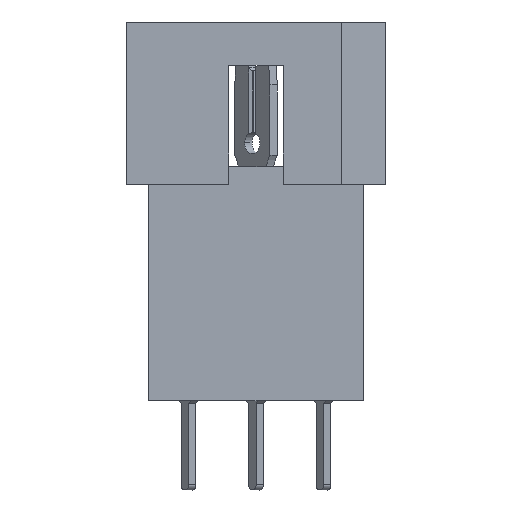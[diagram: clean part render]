
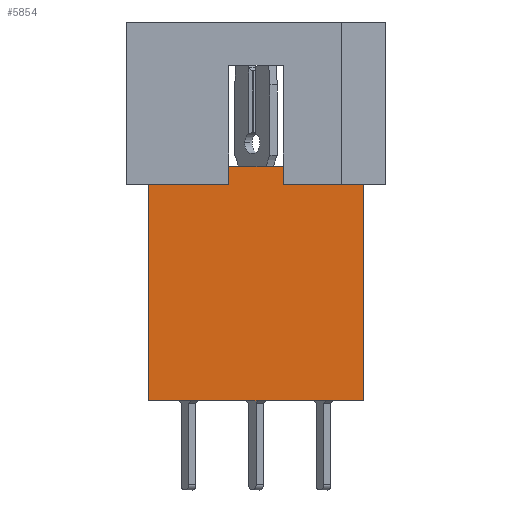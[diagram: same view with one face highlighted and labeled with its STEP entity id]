
A CAD part, top view. The second image highlights one B-rep face of the part: STEP entity #5854.
In plain terms, the highlighted planar face has unit normal (0, 0, 1).
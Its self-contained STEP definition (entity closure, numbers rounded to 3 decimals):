
#20 = CARTESIAN_POINT ( 'NONE',  ( 5.563, 0., 2.54 ) ) ;
#163 = DIRECTION ( 'NONE',  ( 1., 0., 0. ) ) ;
#215 = VECTOR ( 'NONE', #2633, 1000. ) ;
#218 = VECTOR ( 'NONE', #1200, 1000. ) ;
#232 = EDGE_LOOP ( 'NONE', ( #4984, #563, #6303, #2303, #3558, #2815, #1985, #5586 ) ) ;
#261 = VECTOR ( 'NONE', #4432, 1000. ) ;
#319 = CARTESIAN_POINT ( 'NONE',  ( -2.324, 0., 2.54 ) ) ;
#379 = LINE ( 'NONE', #5219, #218 ) ;
#386 = VERTEX_POINT ( 'NONE', #4853 ) ;
#469 = DIRECTION ( 'NONE',  ( 0., -1., 0. ) ) ;
#563 = ORIENTED_EDGE ( 'NONE', *, *, #4137, .F. ) ;
#750 = EDGE_CURVE ( 'NONE', #3537, #2194, #3150, .T. ) ;
#1133 = DIRECTION ( 'NONE',  ( 0., 0., 1. ) ) ;
#1200 = DIRECTION ( 'NONE',  ( 0., 1., 0. ) ) ;
#1385 = DIRECTION ( 'NONE',  ( 1., 0., 0. ) ) ;
#1396 = EDGE_CURVE ( 'NONE', #5002, #4789, #2987, .T. ) ;
#1629 = VECTOR ( 'NONE', #4378, 1000. ) ;
#1632 = CARTESIAN_POINT ( 'NONE',  ( -2.324, 0., 2.54 ) ) ;
#1648 = DIRECTION ( 'NONE',  ( 1., 0., 0. ) ) ;
#1733 = FACE_OUTER_BOUND ( 'NONE', #232, .T. ) ;
#1855 = LINE ( 'NONE', #6491, #2577 ) ;
#1897 = CARTESIAN_POINT ( 'NONE',  ( 2.362, 1.016, 2.54 ) ) ;
#1985 = ORIENTED_EDGE ( 'NONE', *, *, #1396, .F. ) ;
#2143 = PLANE ( 'NONE',  #5382 ) ;
#2194 = VERTEX_POINT ( 'NONE', #3525 ) ;
#2303 = ORIENTED_EDGE ( 'NONE', *, *, #2860, .T. ) ;
#2307 = DIRECTION ( 'NONE',  ( 1., 0., 0. ) ) ;
#2368 = CARTESIAN_POINT ( 'NONE',  ( 5.563, 1.016, 2.54 ) ) ;
#2459 = CARTESIAN_POINT ( 'NONE',  ( 2.362, 6.985, 2.54 ) ) ;
#2577 = VECTOR ( 'NONE', #1385, 1000. ) ;
#2633 = DIRECTION ( 'NONE',  ( 1., 0., 0. ) ) ;
#2815 = ORIENTED_EDGE ( 'NONE', *, *, #6182, .T. ) ;
#2860 = EDGE_CURVE ( 'NONE', #386, #4471, #3284, .T. ) ;
#2987 = LINE ( 'NONE', #5242, #5318 ) ;
#3150 = LINE ( 'NONE', #3621, #215 ) ;
#3270 = EDGE_CURVE ( 'NONE', #4500, #4471, #5161, .T. ) ;
#3284 = LINE ( 'NONE', #6372, #1629 ) ;
#3438 = VECTOR ( 'NONE', #469, 1000. ) ;
#3525 = CARTESIAN_POINT ( 'NONE',  ( 2.362, 0., 2.54 ) ) ;
#3529 = LINE ( 'NONE', #4452, #261 ) ;
#3537 = VERTEX_POINT ( 'NONE', #319 ) ;
#3558 = ORIENTED_EDGE ( 'NONE', *, *, #3270, .F. ) ;
#3621 = CARTESIAN_POINT ( 'NONE',  ( -2.324, 0., 2.54 ) ) ;
#3814 = VECTOR ( 'NONE', #163, 1000. ) ;
#4001 = EDGE_CURVE ( 'NONE', #5247, #386, #1855, .T. ) ;
#4137 = EDGE_CURVE ( 'NONE', #5247, #3537, #3529, .T. ) ;
#4150 = CARTESIAN_POINT ( 'NONE',  ( -2.324, -12.7, 2.54 ) ) ;
#4378 = DIRECTION ( 'NONE',  ( 0., 1., 0. ) ) ;
#4432 = DIRECTION ( 'NONE',  ( 0., 1., 0. ) ) ;
#4452 = CARTESIAN_POINT ( 'NONE',  ( -2.324, -12.7, 2.54 ) ) ;
#4471 = VERTEX_POINT ( 'NONE', #6027 ) ;
#4500 = VERTEX_POINT ( 'NONE', #20 ) ;
#4595 = CARTESIAN_POINT ( 'NONE',  ( -2.324, -12.7, 2.54 ) ) ;
#4789 = VERTEX_POINT ( 'NONE', #2368 ) ;
#4837 = EDGE_CURVE ( 'NONE', #5002, #2194, #5086, .T. ) ;
#4853 = CARTESIAN_POINT ( 'NONE',  ( 10.249, -12.7, 2.54 ) ) ;
#4984 = ORIENTED_EDGE ( 'NONE', *, *, #750, .F. ) ;
#5002 = VERTEX_POINT ( 'NONE', #1897 ) ;
#5086 = LINE ( 'NONE', #2459, #3438 ) ;
#5161 = LINE ( 'NONE', #1632, #3814 ) ;
#5219 = CARTESIAN_POINT ( 'NONE',  ( 5.563, 6.985, 2.54 ) ) ;
#5242 = CARTESIAN_POINT ( 'NONE',  ( 0., 1.016, 2.54 ) ) ;
#5247 = VERTEX_POINT ( 'NONE', #4595 ) ;
#5318 = VECTOR ( 'NONE', #2307, 1000. ) ;
#5382 = AXIS2_PLACEMENT_3D ( 'NONE', #4150, #1133, #1648 ) ;
#5586 = ORIENTED_EDGE ( 'NONE', *, *, #4837, .T. ) ;
#5854 = ADVANCED_FACE ( 'NONE', ( #1733 ), #2143, .T. ) ;
#6027 = CARTESIAN_POINT ( 'NONE',  ( 10.249, 0., 2.54 ) ) ;
#6182 = EDGE_CURVE ( 'NONE', #4500, #4789, #379, .T. ) ;
#6303 = ORIENTED_EDGE ( 'NONE', *, *, #4001, .T. ) ;
#6372 = CARTESIAN_POINT ( 'NONE',  ( 10.249, -12.7, 2.54 ) ) ;
#6491 = CARTESIAN_POINT ( 'NONE',  ( -2.324, -12.7, 2.54 ) ) ;
